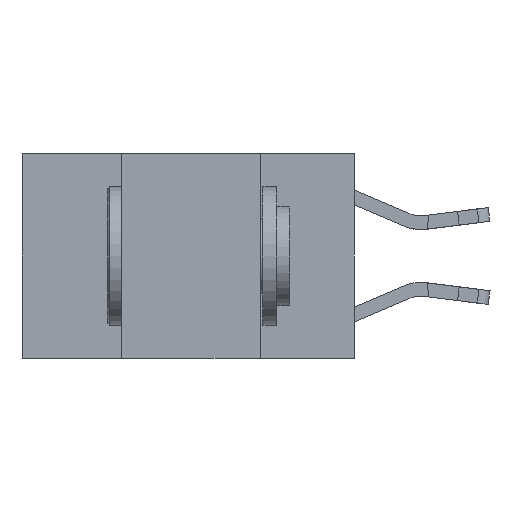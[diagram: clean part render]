
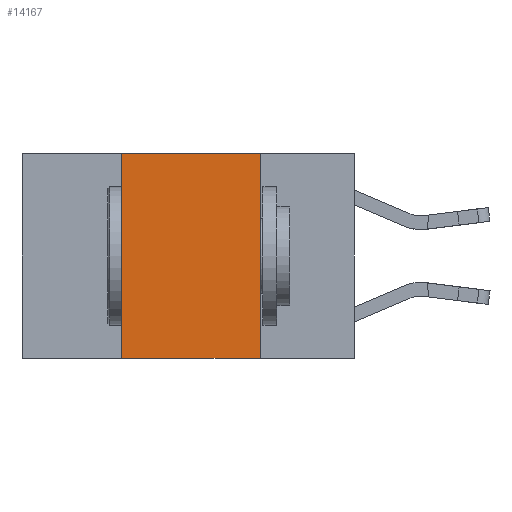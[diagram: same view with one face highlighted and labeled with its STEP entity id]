
A CAD part, left-side view. The second image highlights one B-rep face of the part: STEP entity #14167.
In plain terms, the highlighted planar face has unit normal (-1, 0, 0).
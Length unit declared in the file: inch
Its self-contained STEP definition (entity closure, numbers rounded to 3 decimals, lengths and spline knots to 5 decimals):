
#464 = LINE ( 'NONE', #1607, #8614 ) ;
#647 = EDGE_LOOP ( 'NONE', ( #18910, #2342, #15182, #7675 ) ) ;
#1607 = CARTESIAN_POINT ( 'NONE',  ( 0., 0.6, 0. ) ) ;
#2103 = LINE ( 'NONE', #13422, #5908 ) ;
#2342 = ORIENTED_EDGE ( 'NONE', *, *, #8165, .F. ) ;
#2552 = VECTOR ( 'NONE', #3496, 39.37008 ) ;
#3256 = DIRECTION ( 'NONE',  ( 0., -1., 0. ) ) ;
#3496 = DIRECTION ( 'NONE',  ( 0., -1., 0. ) ) ;
#4879 = CARTESIAN_POINT ( 'NONE',  ( 0., 0.42, -0.37 ) ) ;
#5908 = VECTOR ( 'NONE', #15028, 39.37008 ) ;
#6249 = CARTESIAN_POINT ( 'NONE',  ( 0., 0.6, 0. ) ) ;
#6709 = CARTESIAN_POINT ( 'NONE',  ( 0., 0.17, 0. ) ) ;
#7571 = EDGE_CURVE ( 'NONE', #8185, #18996, #7873, .T. ) ;
#7675 = ORIENTED_EDGE ( 'NONE', *, *, #7571, .T. ) ;
#7873 = LINE ( 'NONE', #9905, #2552 ) ;
#8165 = EDGE_CURVE ( 'NONE', #17005, #17271, #464, .T. ) ;
#8185 = VERTEX_POINT ( 'NONE', #4879 ) ;
#8614 = VECTOR ( 'NONE', #3256, 39.37008 ) ;
#9474 = DIRECTION ( 'NONE',  ( 0., 0., -1. ) ) ;
#9905 = CARTESIAN_POINT ( 'NONE',  ( 0., 0.6, -0.37 ) ) ;
#10848 = FACE_OUTER_BOUND ( 'NONE', #647, .T. ) ;
#11858 = EDGE_CURVE ( 'NONE', #8185, #17005, #2103, .T. ) ;
#12815 = CARTESIAN_POINT ( 'NONE',  ( 0., 0.17, -0.37 ) ) ;
#12941 = EDGE_CURVE ( 'NONE', #17271, #18996, #15924, .T. ) ;
#13422 = CARTESIAN_POINT ( 'NONE',  ( 0., 0.42, 0. ) ) ;
#14167 = ADVANCED_FACE ( 'NONE', ( #10848 ), #15848, .F. ) ;
#15028 = DIRECTION ( 'NONE',  ( 0., 0., 1. ) ) ;
#15182 = ORIENTED_EDGE ( 'NONE', *, *, #11858, .F. ) ;
#15848 = PLANE ( 'NONE',  #17499 ) ;
#15924 = LINE ( 'NONE', #6709, #19637 ) ;
#16302 = DIRECTION ( 'NONE',  ( 0., 0., -1. ) ) ;
#16308 = CARTESIAN_POINT ( 'NONE',  ( 0., 0.17, 0. ) ) ;
#17005 = VERTEX_POINT ( 'NONE', #18888 ) ;
#17271 = VERTEX_POINT ( 'NONE', #16308 ) ;
#17499 = AXIS2_PLACEMENT_3D ( 'NONE', #6249, #19040, #9474 ) ;
#18888 = CARTESIAN_POINT ( 'NONE',  ( 0., 0.42, 0. ) ) ;
#18910 = ORIENTED_EDGE ( 'NONE', *, *, #12941, .F. ) ;
#18996 = VERTEX_POINT ( 'NONE', #12815 ) ;
#19040 = DIRECTION ( 'NONE',  ( 1., 0., 0. ) ) ;
#19637 = VECTOR ( 'NONE', #16302, 39.37008 ) ;
